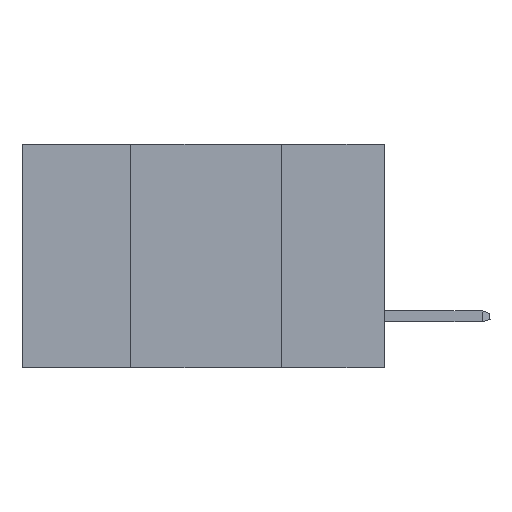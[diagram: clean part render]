
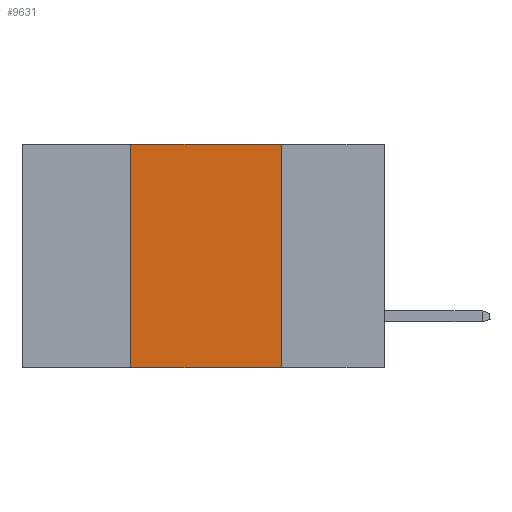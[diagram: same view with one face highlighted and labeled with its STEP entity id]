
A CAD part, left-side view. The second image highlights one B-rep face of the part: STEP entity #9631.
In plain terms, the highlighted planar face has unit normal (-1, 0, 0).
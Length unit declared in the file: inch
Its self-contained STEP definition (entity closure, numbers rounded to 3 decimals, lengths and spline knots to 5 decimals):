
#294 = CARTESIAN_POINT ( 'NONE',  ( 0., 0.42, 0. ) ) ;
#976 = VERTEX_POINT ( 'NONE', #4766 ) ;
#1746 = LINE ( 'NONE', #294, #5627 ) ;
#2364 = EDGE_CURVE ( 'NONE', #11927, #9452, #1746, .T. ) ;
#3137 = DIRECTION ( 'NONE',  ( 0., 0., -1. ) ) ;
#3180 = EDGE_CURVE ( 'NONE', #11927, #9990, #17840, .T. ) ;
#3533 = EDGE_LOOP ( 'NONE', ( #14164, #9880, #8970, #13570 ) ) ;
#3715 = LINE ( 'NONE', #4239, #4756 ) ;
#3791 = PLANE ( 'NONE',  #11127 ) ;
#3858 = CARTESIAN_POINT ( 'NONE',  ( 0., 0.6, 0. ) ) ;
#4239 = CARTESIAN_POINT ( 'NONE',  ( 0., 0.6, 0. ) ) ;
#4756 = VECTOR ( 'NONE', #17345, 39.37008 ) ;
#4766 = CARTESIAN_POINT ( 'NONE',  ( 0., 0.17, 0. ) ) ;
#5530 = DIRECTION ( 'NONE',  ( 0., 0., -1. ) ) ;
#5627 = VECTOR ( 'NONE', #20405, 39.37008 ) ;
#6278 = CARTESIAN_POINT ( 'NONE',  ( 0., 0.17, 0. ) ) ;
#7307 = VECTOR ( 'NONE', #3137, 39.37008 ) ;
#8970 = ORIENTED_EDGE ( 'NONE', *, *, #2364, .F. ) ;
#9452 = VERTEX_POINT ( 'NONE', #13632 ) ;
#9631 = ADVANCED_FACE ( 'NONE', ( #9951 ), #3791, .F. ) ;
#9880 = ORIENTED_EDGE ( 'NONE', *, *, #13797, .F. ) ;
#9951 = FACE_OUTER_BOUND ( 'NONE', #3533, .T. ) ;
#9990 = VERTEX_POINT ( 'NONE', #13370 ) ;
#10365 = EDGE_CURVE ( 'NONE', #976, #9990, #16644, .T. ) ;
#11127 = AXIS2_PLACEMENT_3D ( 'NONE', #3858, #15498, #5530 ) ;
#11927 = VERTEX_POINT ( 'NONE', #21580 ) ;
#12883 = CARTESIAN_POINT ( 'NONE',  ( 0., 0.6, -0.37 ) ) ;
#13324 = DIRECTION ( 'NONE',  ( 0., -1., 0. ) ) ;
#13370 = CARTESIAN_POINT ( 'NONE',  ( 0., 0.17, -0.37 ) ) ;
#13570 = ORIENTED_EDGE ( 'NONE', *, *, #3180, .T. ) ;
#13632 = CARTESIAN_POINT ( 'NONE',  ( 0., 0.42, 0. ) ) ;
#13797 = EDGE_CURVE ( 'NONE', #9452, #976, #3715, .T. ) ;
#14164 = ORIENTED_EDGE ( 'NONE', *, *, #10365, .F. ) ;
#14676 = VECTOR ( 'NONE', #13324, 39.37008 ) ;
#15498 = DIRECTION ( 'NONE',  ( 1., 0., 0. ) ) ;
#16644 = LINE ( 'NONE', #6278, #7307 ) ;
#17345 = DIRECTION ( 'NONE',  ( 0., -1., 0. ) ) ;
#17840 = LINE ( 'NONE', #12883, #14676 ) ;
#20405 = DIRECTION ( 'NONE',  ( 0., 0., 1. ) ) ;
#21580 = CARTESIAN_POINT ( 'NONE',  ( 0., 0.42, -0.37 ) ) ;
